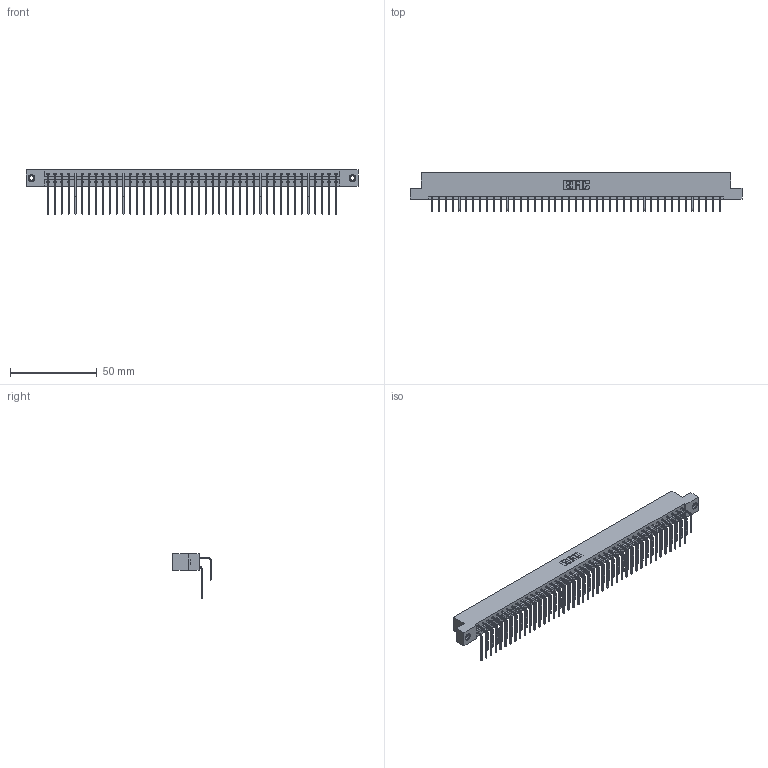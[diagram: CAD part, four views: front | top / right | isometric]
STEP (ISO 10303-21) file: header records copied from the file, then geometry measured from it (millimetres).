
FILE_DESCRIPTION (( 'STEP AP203' ), '1' );
FILE_NAME ('833-086-558-207.STEP', '2020-06-06T04:09:01', ( '' ), ( '' ), 'SwSTEP 2.0', 'SolidWorks 2020', '' );
FILE_SCHEMA (( 'CONFIG_CONTROL_DESIGN' ));
Length unit declared in the file: inch
Products named in the file (5): 345-250-001_345-250-005-103; 345-292-001_558 559 Tail - 1; 833 Part_Flush - .156 Dia - TI; 833-086-558-207; 345-292-001_558 Tail - 2
Assembly tree (89 placements, depth 2):
  833-086-558-207
    833 Part_Flush - .156 Dia - TI
    345-292-001_558 559 Tail - 1  x43
    345-292-001_558 Tail - 2  x43
    345-250-001_345-250-005-103  x2
Bounding box: 191.92 x 22.17 x 25.53 mm (x, y, z)
Volume: 20086.1 mm3; surface area: 26262.8 mm2
Topology: 89 solids, 89 shells, 4818 faces, 14293 edges, 9406 vertices
Faces by surface type: plane 3370, cylinder 1432, cone 12, torus 4
Entity records: 30504 total; most frequent: CARTESIAN_POINT 5088, ORIENTED_EDGE 4966, DIRECTION 4357, EDGE_CURVE 2483, VECTOR 2295, LINE 2295, VERTEX_POINT 1648, AXIS2_PLACEMENT_3D 1031
